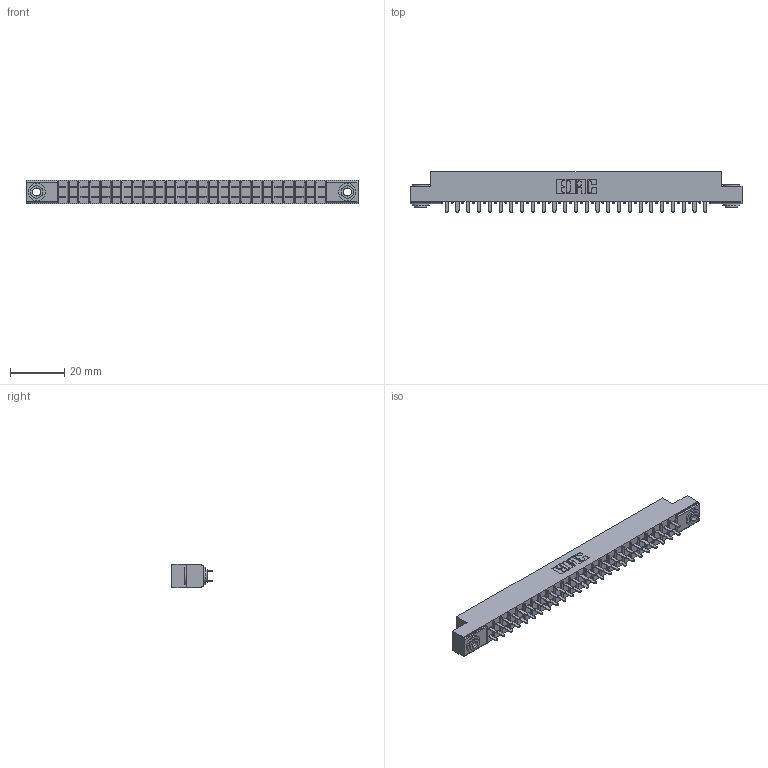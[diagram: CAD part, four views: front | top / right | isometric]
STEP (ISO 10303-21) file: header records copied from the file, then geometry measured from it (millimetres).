
FILE_DESCRIPTION (( 'STEP AP203' ), '1' );
FILE_NAME ('315-050-521-203.STEP', '2019-09-10T18:41:43', ( '' ), ( '' ), 'SwSTEP 2.0', 'SolidWorks 2016', '' );
FILE_SCHEMA (( 'CONFIG_CONTROL_DESIGN' ));
Length unit declared in the file: inch
Products named in the file (4): 305 Part_.156 Dia; 315-050-521-203; 345-250-002_345-250-002-102; 305-290-001_521
Assembly tree (53 placements, depth 2):
  315-050-521-203
    305 Part_.156 Dia
    305-290-001_521  x50
    345-250-002_345-250-002-102  x2
Bounding box: 122.07 x 14.86 x 8.71 mm (x, y, z)
Volume: 7610.3 mm3; surface area: 14572.4 mm2
Topology: 53 solids, 53 shells, 2468 faces, 7003 edges, 4530 vertices
Faces by surface type: plane 1442, cylinder 918, sphere 100, cone 8
Entity records: 30083 total; most frequent: CARTESIAN_POINT 4958, ORIENTED_EDGE 4910, DIRECTION 4825, EDGE_CURVE 2455, LINE 1959, VECTOR 1959, VERTEX_POINT 1566, AXIS2_PLACEMENT_3D 1433
